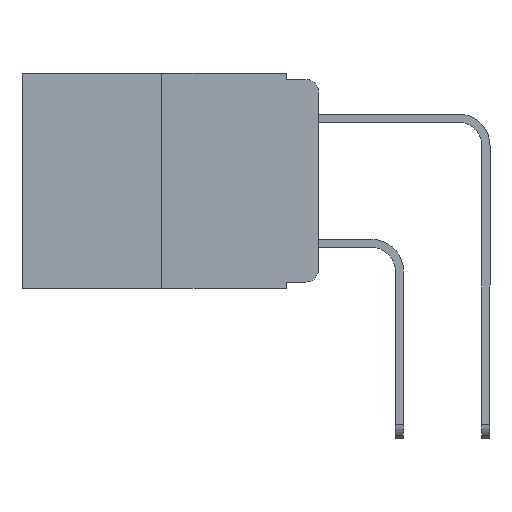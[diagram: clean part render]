
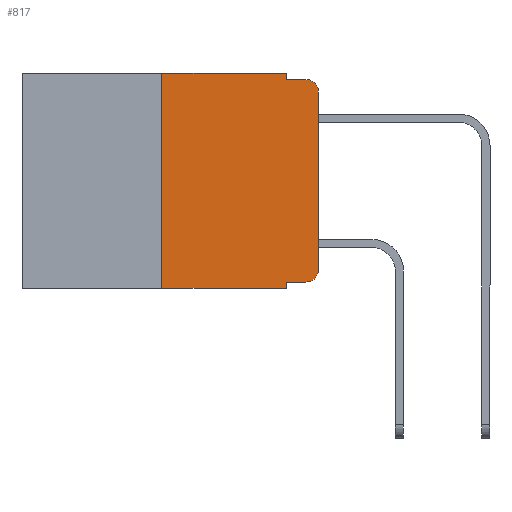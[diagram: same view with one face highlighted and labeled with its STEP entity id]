
A CAD part, left-side view. The second image highlights one B-rep face of the part: STEP entity #817.
In plain terms, the highlighted planar face has unit normal (-1, 0, 0).
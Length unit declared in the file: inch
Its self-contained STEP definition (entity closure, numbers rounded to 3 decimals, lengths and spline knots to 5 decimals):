
#80 = VECTOR ( 'NONE', #5249, 39.37008 ) ;
#509 = CARTESIAN_POINT ( 'NONE',  ( 0., 0.25, 0. ) ) ;
#522 = DIRECTION ( 'NONE',  ( 0., 0., -1. ) ) ;
#593 = CARTESIAN_POINT ( 'NONE',  ( 0., 0.051, -0.01 ) ) ;
#754 = ORIENTED_EDGE ( 'NONE', *, *, #1889, .F. ) ;
#815 = VERTEX_POINT ( 'NONE', #7710 ) ;
#817 = ADVANCED_FACE ( 'NONE', ( #4289 ), #7308, .F. ) ;
#998 = DIRECTION ( 'NONE',  ( 0., 0., -1. ) ) ;
#1059 = AXIS2_PLACEMENT_3D ( 'NONE', #7236, #7255, #7435 ) ;
#1220 = CARTESIAN_POINT ( 'NONE',  ( 0., 0.051, 0. ) ) ;
#1525 = EDGE_CURVE ( 'NONE', #5162, #6615, #8777, .T. ) ;
#1641 = DIRECTION ( 'NONE',  ( 0., 0., 1. ) ) ;
#1642 = EDGE_LOOP ( 'NONE', ( #9375, #9588, #754, #3647, #6125, #3962, #6372, #10260, #8587, #10487 ) ) ;
#1718 = EDGE_CURVE ( 'NONE', #1974, #5716, #9665, .T. ) ;
#1870 = EDGE_CURVE ( 'NONE', #10023, #815, #9338, .T. ) ;
#1887 = EDGE_CURVE ( 'NONE', #815, #6495, #7161, .T. ) ;
#1889 = EDGE_CURVE ( 'NONE', #8130, #6495, #5284, .T. ) ;
#1906 = EDGE_CURVE ( 'NONE', #6615, #8130, #8879, .T. ) ;
#1907 = EDGE_CURVE ( 'NONE', #1974, #5162, #6079, .T. ) ;
#1908 = EDGE_CURVE ( 'NONE', #6549, #5716, #4681, .T. ) ;
#1923 = EDGE_CURVE ( 'NONE', #6549, #7519, #4361, .T. ) ;
#1926 = EDGE_CURVE ( 'NONE', #7519, #10023, #2074, .T. ) ;
#1974 = VERTEX_POINT ( 'NONE', #3626 ) ;
#2074 = CIRCLE ( 'NONE', #7357, 0.02 ) ;
#2113 = CARTESIAN_POINT ( 'NONE',  ( 0., 0.051, -0.343 ) ) ;
#2379 = VECTOR ( 'NONE', #6611, 39.37008 ) ;
#2702 = VECTOR ( 'NONE', #6320, 39.37008 ) ;
#3159 = VECTOR ( 'NONE', #8484, 39.37008 ) ;
#3626 = CARTESIAN_POINT ( 'NONE',  ( 0., 0.25, -0.343 ) ) ;
#3647 = ORIENTED_EDGE ( 'NONE', *, *, #1906, .F. ) ;
#3962 = ORIENTED_EDGE ( 'NONE', *, *, #1907, .F. ) ;
#4176 = CARTESIAN_POINT ( 'NONE',  ( 0., 0.02, -0.333 ) ) ;
#4289 = FACE_OUTER_BOUND ( 'NONE', #1642, .T. ) ;
#4361 = LINE ( 'NONE', #5252, #80 ) ;
#4592 = CARTESIAN_POINT ( 'NONE',  ( 0., 0.051, 0. ) ) ;
#4681 = LINE ( 'NONE', #1220, #10545 ) ;
#4995 = CARTESIAN_POINT ( 'NONE',  ( 0., 0.25, 0. ) ) ;
#5162 = VERTEX_POINT ( 'NONE', #4995 ) ;
#5249 = DIRECTION ( 'NONE',  ( 0., -1., 0. ) ) ;
#5252 = CARTESIAN_POINT ( 'NONE',  ( 0., 0.051, -0.333 ) ) ;
#5284 = LINE ( 'NONE', #6559, #2379 ) ;
#5474 = CARTESIAN_POINT ( 'NONE',  ( 0., 0.051, 0. ) ) ;
#5475 = CARTESIAN_POINT ( 'NONE',  ( 0., 0.051, -0.333 ) ) ;
#5592 = CARTESIAN_POINT ( 'NONE',  ( 0., 0., 0. ) ) ;
#5716 = VERTEX_POINT ( 'NONE', #2113 ) ;
#5912 = CARTESIAN_POINT ( 'NONE',  ( 0., 0.02, -0.03 ) ) ;
#5933 = DIRECTION ( 'NONE',  ( 0., 0., -1. ) ) ;
#5948 = DIRECTION ( 'NONE',  ( -1., 0., 0. ) ) ;
#6043 = DIRECTION ( 'NONE',  ( 0., 0., -1. ) ) ;
#6078 = DIRECTION ( 'NONE',  ( -1., 0., 0. ) ) ;
#6079 = LINE ( 'NONE', #509, #10767 ) ;
#6125 = ORIENTED_EDGE ( 'NONE', *, *, #1525, .F. ) ;
#6320 = DIRECTION ( 'NONE',  ( 0., 0., 1. ) ) ;
#6344 = AXIS2_PLACEMENT_3D ( 'NONE', #5912, #6078, #6043 ) ;
#6372 = ORIENTED_EDGE ( 'NONE', *, *, #1718, .T. ) ;
#6490 = CARTESIAN_POINT ( 'NONE',  ( 0., 0.02, -0.313 ) ) ;
#6495 = VERTEX_POINT ( 'NONE', #7817 ) ;
#6549 = VERTEX_POINT ( 'NONE', #5475 ) ;
#6559 = CARTESIAN_POINT ( 'NONE',  ( 0., 0.051, -0.01 ) ) ;
#6611 = DIRECTION ( 'NONE',  ( 0., -1., 0. ) ) ;
#6615 = VERTEX_POINT ( 'NONE', #4592 ) ;
#6932 = VECTOR ( 'NONE', #522, 39.37008 ) ;
#7161 = CIRCLE ( 'NONE', #6344, 0.02 ) ;
#7236 = CARTESIAN_POINT ( 'NONE',  ( 0., 0.473, 0. ) ) ;
#7255 = DIRECTION ( 'NONE',  ( 1., 0., 0. ) ) ;
#7308 = PLANE ( 'NONE',  #1059 ) ;
#7357 = AXIS2_PLACEMENT_3D ( 'NONE', #6490, #5948, #5933 ) ;
#7435 = DIRECTION ( 'NONE',  ( 0., 0., -1. ) ) ;
#7519 = VERTEX_POINT ( 'NONE', #4176 ) ;
#7541 = CARTESIAN_POINT ( 'NONE',  ( 0., 0., -0.313 ) ) ;
#7710 = CARTESIAN_POINT ( 'NONE',  ( 0., 0., -0.03 ) ) ;
#7817 = CARTESIAN_POINT ( 'NONE',  ( 0., 0.02, -0.01 ) ) ;
#8130 = VERTEX_POINT ( 'NONE', #593 ) ;
#8484 = DIRECTION ( 'NONE',  ( 0., -1., 0. ) ) ;
#8555 = CARTESIAN_POINT ( 'NONE',  ( 0., 0.473, -0.343 ) ) ;
#8587 = ORIENTED_EDGE ( 'NONE', *, *, #1923, .T. ) ;
#8777 = LINE ( 'NONE', #9972, #10890 ) ;
#8879 = LINE ( 'NONE', #5474, #6932 ) ;
#9338 = LINE ( 'NONE', #5592, #2702 ) ;
#9375 = ORIENTED_EDGE ( 'NONE', *, *, #1870, .T. ) ;
#9588 = ORIENTED_EDGE ( 'NONE', *, *, #1887, .T. ) ;
#9665 = LINE ( 'NONE', #8555, #3159 ) ;
#9949 = DIRECTION ( 'NONE',  ( 0., -1., 0. ) ) ;
#9972 = CARTESIAN_POINT ( 'NONE',  ( 0., 0.473, 0. ) ) ;
#10023 = VERTEX_POINT ( 'NONE', #7541 ) ;
#10260 = ORIENTED_EDGE ( 'NONE', *, *, #1908, .F. ) ;
#10487 = ORIENTED_EDGE ( 'NONE', *, *, #1926, .T. ) ;
#10545 = VECTOR ( 'NONE', #998, 39.37008 ) ;
#10767 = VECTOR ( 'NONE', #1641, 39.37008 ) ;
#10890 = VECTOR ( 'NONE', #9949, 39.37008 ) ;
